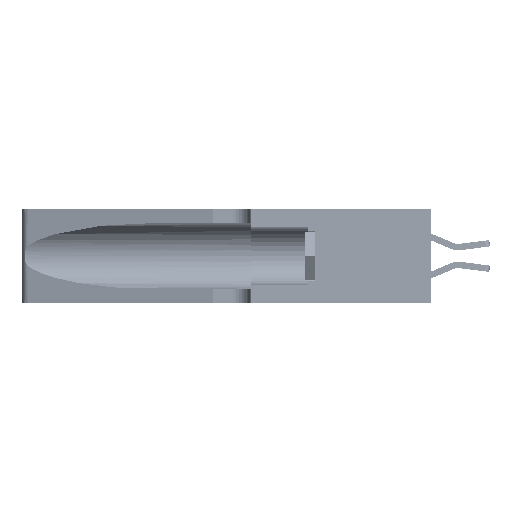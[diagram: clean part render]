
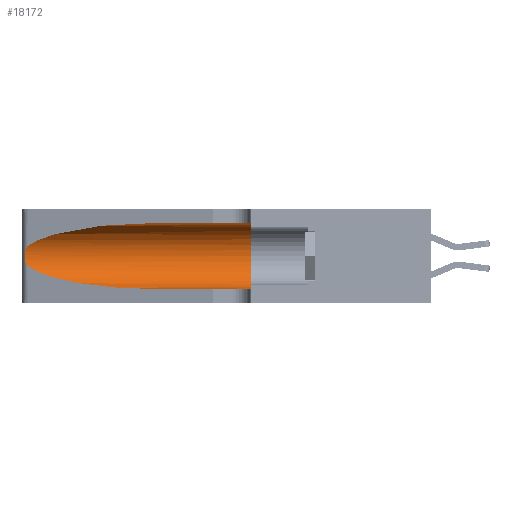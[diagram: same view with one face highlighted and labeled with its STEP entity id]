
A CAD part, left-side view. The second image highlights one B-rep face of the part: STEP entity #18172.
In plain terms, the highlighted cylindrical face has radius 3.308 mm (diameter 6.617 mm), a partial arc.
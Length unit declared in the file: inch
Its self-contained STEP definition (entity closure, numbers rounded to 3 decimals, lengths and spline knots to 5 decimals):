
#113 = CARTESIAN_POINT ( 'NONE',  ( 0.25639, 1.23186, 0.15144 ) ) ;
#260 = CARTESIAN_POINT ( 'NONE',  ( 0.1305, 0.35, 0.185 ) ) ;
#665 = CARTESIAN_POINT ( 'NONE',  ( 0.1305, 0.72297, 0.31525 ) ) ;
#1076 = CARTESIAN_POINT ( 'NONE',  ( 0.1305, 1.61858, 0.31525 ) ) ;
#3020 = VERTEX_POINT ( 'NONE', #39976 ) ;
#3668 = EDGE_CURVE ( 'NONE', #3020, #5633, #17796, .T. ) ;
#3767 = ORIENTED_EDGE ( 'NONE', *, *, #6647, .T. ) ;
#4430 = CARTESIAN_POINT ( 'NONE',  ( 0.25487, 1.22718, 0.14631 ) ) ;
#4555 = EDGE_CURVE ( 'NONE', #35979, #11805, #13330, .T. ) ;
#5073 =( BOUNDED_CURVE ( )  B_SPLINE_CURVE ( 3, ( #665, #7381, #10740, #27662 ),
 .UNSPECIFIED., .F., .F. ) 
 B_SPLINE_CURVE_WITH_KNOTS ( ( 4, 4 ),
 ( 1.5708, 2.84003 ),
 .UNSPECIFIED. ) 
 CURVE ( )  GEOMETRIC_REPRESENTATION_ITEM ( )  RATIONAL_B_SPLINE_CURVE ( ( 1., 0.87, 0.87, 1. ) ) 
 REPRESENTATION_ITEM ( '' )  );
#5633 = VERTEX_POINT ( 'NONE', #31282 ) ;
#6105 = CARTESIAN_POINT ( 'NONE',  ( 0.26075, 1.23896, 0.19203 ) ) ;
#6647 = EDGE_CURVE ( 'NONE', #34233, #35220, #5073, .T. ) ;
#7381 = CARTESIAN_POINT ( 'NONE',  ( 0.18966, 0.96281, 0.31525 ) ) ;
#7879 = CARTESIAN_POINT ( 'NONE',  ( 0.1305, 0.35, 0.05475 ) ) ;
#7957 = EDGE_CURVE ( 'NONE', #35220, #3020, #26589, .T. ) ;
#9915 = CARTESIAN_POINT ( 'NONE',  ( 0.25487, 1.22718, 0.22369 ) ) ;
#10367 = DIRECTION ( 'NONE',  ( 0., 1., 0. ) ) ;
#10740 = CARTESIAN_POINT ( 'NONE',  ( 0.2373, 1.15595, 0.28018 ) ) ;
#11010 = CARTESIAN_POINT ( 'NONE',  ( 0.1305, 1.61858, 0.185 ) ) ;
#11805 = VERTEX_POINT ( 'NONE', #7879 ) ;
#11967 = LINE ( 'NONE', #1076, #28299 ) ;
#12847 = ORIENTED_EDGE ( 'NONE', *, *, #28117, .T. ) ;
#13161 = CARTESIAN_POINT ( 'NONE',  ( 0.25487, 1.22718, 0.14631 ) ) ;
#13305 = CARTESIAN_POINT ( 'NONE',  ( 0.26017, 1.23833, 0.17102 ) ) ;
#13330 = CIRCLE ( 'NONE', #15001, 0.13025 ) ;
#13778 = CYLINDRICAL_SURFACE ( 'NONE', #32175, 0.13025 ) ;
#15001 = AXIS2_PLACEMENT_3D ( 'NONE', #260, #10367, #37502 ) ;
#15475 = ORIENTED_EDGE ( 'NONE', *, *, #4555, .F. ) ;
#16232 = CARTESIAN_POINT ( 'NONE',  ( 0.25787, 1.23484, 0.2124 ) ) ;
#16699 = CARTESIAN_POINT ( 'NONE',  ( 0.25555, 1.22993, 0.14849 ) ) ;
#17796 =( BOUNDED_CURVE ( )  B_SPLINE_CURVE ( 3, ( #4430, #18237, #34506, #41499 ),
 .UNSPECIFIED., .F., .T. ) 
 B_SPLINE_CURVE_WITH_KNOTS ( ( 4, 4 ),
 ( 3.44316, 4.71239 ),
 .UNSPECIFIED. ) 
 CURVE ( )  GEOMETRIC_REPRESENTATION_ITEM ( )  RATIONAL_B_SPLINE_CURVE ( ( 1., 0.87, 0.87, 1. ) ) 
 REPRESENTATION_ITEM ( '' )  );
#18172 = ADVANCED_FACE ( 'NONE', ( #40489 ), #13778, .F. ) ;
#18237 = CARTESIAN_POINT ( 'NONE',  ( 0.2373, 1.15595, 0.08982 ) ) ;
#18540 = CARTESIAN_POINT ( 'NONE',  ( 0.1305, 0.35, 0.31525 ) ) ;
#19542 = LINE ( 'NONE', #32524, #36328 ) ;
#22163 = DIRECTION ( 'NONE',  ( 0., -1., 0. ) ) ;
#22182 = CARTESIAN_POINT ( 'NONE',  ( 0.25487, 1.22718, 0.22369 ) ) ;
#24161 = ORIENTED_EDGE ( 'NONE', *, *, #3668, .T. ) ;
#25778 = ORIENTED_EDGE ( 'NONE', *, *, #7957, .T. ) ;
#26224 = CARTESIAN_POINT ( 'NONE',  ( 0.25555, 1.22994, 0.2215 ) ) ;
#26527 = CARTESIAN_POINT ( 'NONE',  ( 0.26075, 1.23896, 0.178 ) ) ;
#26589 = B_SPLINE_CURVE_WITH_KNOTS ( 'NONE', 3,
 ( #9915, #26224, #43193, #16232, #33411, #33114, #6105, #26527, #13305, #33267, #30178, #113, #16699, #13161 ),
 .UNSPECIFIED., .F., .F.,
 ( 4, 2, 2, 2, 2, 2, 4 ),
 ( 0., 0.00027, 0.00053, 0.00107, 0.0016, 0.00187, 0.00214 ),
 .UNSPECIFIED. ) ;
#26692 = CARTESIAN_POINT ( 'NONE',  ( 0.1305, 0.72297, 0.31525 ) ) ;
#27662 = CARTESIAN_POINT ( 'NONE',  ( 0.25487, 1.22718, 0.22369 ) ) ;
#28117 = EDGE_CURVE ( 'NONE', #5633, #11805, #19542, .T. ) ;
#28299 = VECTOR ( 'NONE', #34495, 39.37008 ) ;
#28481 = ORIENTED_EDGE ( 'NONE', *, *, #36418, .F. ) ;
#28773 = DIRECTION ( 'NONE',  ( 0., 0., -1. ) ) ;
#29579 = DIRECTION ( 'NONE',  ( 0., -1., 0. ) ) ;
#30178 = CARTESIAN_POINT ( 'NONE',  ( 0.25789, 1.23486, 0.15765 ) ) ;
#31282 = CARTESIAN_POINT ( 'NONE',  ( 0.1305, 0.72297, 0.05475 ) ) ;
#32175 = AXIS2_PLACEMENT_3D ( 'NONE', #11010, #22163, #28773 ) ;
#32524 = CARTESIAN_POINT ( 'NONE',  ( 0.1305, 1.61858, 0.05475 ) ) ;
#32946 = EDGE_LOOP ( 'NONE', ( #3767, #25778, #24161, #12847, #15475, #28481 ) ) ;
#33114 = CARTESIAN_POINT ( 'NONE',  ( 0.26018, 1.23835, 0.19895 ) ) ;
#33267 = CARTESIAN_POINT ( 'NONE',  ( 0.25856, 1.23593, 0.16098 ) ) ;
#33411 = CARTESIAN_POINT ( 'NONE',  ( 0.25854, 1.2359, 0.20912 ) ) ;
#34233 = VERTEX_POINT ( 'NONE', #26692 ) ;
#34495 = DIRECTION ( 'NONE',  ( 0., -1., 0. ) ) ;
#34506 = CARTESIAN_POINT ( 'NONE',  ( 0.18966, 0.96281, 0.05475 ) ) ;
#35220 = VERTEX_POINT ( 'NONE', #22182 ) ;
#35979 = VERTEX_POINT ( 'NONE', #18540 ) ;
#36328 = VECTOR ( 'NONE', #29579, 39.37008 ) ;
#36418 = EDGE_CURVE ( 'NONE', #34233, #35979, #11967, .T. ) ;
#37502 = DIRECTION ( 'NONE',  ( 0., 0., 1. ) ) ;
#39976 = CARTESIAN_POINT ( 'NONE',  ( 0.25487, 1.22718, 0.14631 ) ) ;
#40489 = FACE_OUTER_BOUND ( 'NONE', #32946, .T. ) ;
#41499 = CARTESIAN_POINT ( 'NONE',  ( 0.1305, 0.72297, 0.05475 ) ) ;
#43193 = CARTESIAN_POINT ( 'NONE',  ( 0.25639, 1.23184, 0.21858 ) ) ;
